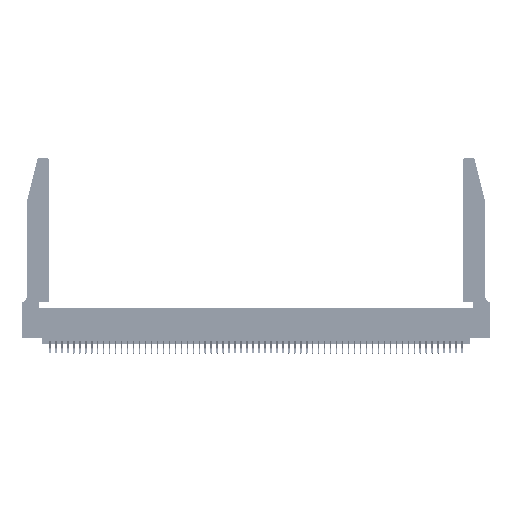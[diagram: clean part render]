
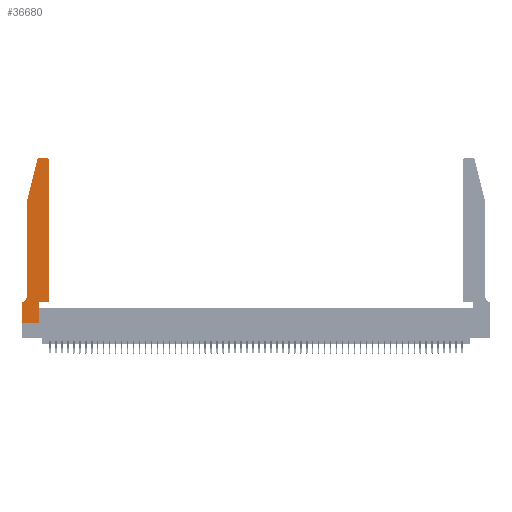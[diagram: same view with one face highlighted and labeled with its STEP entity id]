
A CAD part, top view. The second image highlights one B-rep face of the part: STEP entity #36680.
In plain terms, the highlighted planar face has unit normal (0, 0, 1).
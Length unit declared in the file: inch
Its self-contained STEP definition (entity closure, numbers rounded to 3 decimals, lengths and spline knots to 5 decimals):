
#419 = LINE ( 'NONE', #42385, #19449 ) ;
#731 = VERTEX_POINT ( 'NONE', #7288 ) ;
#1099 = CARTESIAN_POINT ( 'NONE',  ( 0.2865, 0.35, 0.37 ) ) ;
#2258 = LINE ( 'NONE', #23339, #9062 ) ;
#2402 = VERTEX_POINT ( 'NONE', #34915 ) ;
#2714 = CARTESIAN_POINT ( 'NONE',  ( 0.4205, 2.72, 0.37 ) ) ;
#3267 = EDGE_LOOP ( 'NONE', ( #22758, #41664, #4984, #45784, #14533, #25274, #8740, #31765, #51110, #8855, #9467, #22605 ) ) ;
#3878 = VECTOR ( 'NONE', #18521, 39.37008 ) ;
#4937 = LINE ( 'NONE', #1099, #11711 ) ;
#4984 = ORIENTED_EDGE ( 'NONE', *, *, #9804, .T. ) ;
#5143 = EDGE_CURVE ( 'NONE', #15108, #14876, #2258, .T. ) ;
#5638 = LINE ( 'NONE', #22326, #36915 ) ;
#5743 = EDGE_CURVE ( 'NONE', #42289, #31634, #5638, .T. ) ;
#6304 = AXIS2_PLACEMENT_3D ( 'NONE', #19725, #20277, #24291 ) ;
#7288 = CARTESIAN_POINT ( 'NONE',  ( 0.4505, 2.72, 0.37 ) ) ;
#7541 = DIRECTION ( 'NONE',  ( -0.239, -0.971, 0. ) ) ;
#7626 = CARTESIAN_POINT ( 'NONE',  ( 0.2865, 0., 0.37 ) ) ;
#7934 = AXIS2_PLACEMENT_3D ( 'NONE', #2714, #42114, #54968 ) ;
#8740 = ORIENTED_EDGE ( 'NONE', *, *, #15835, .T. ) ;
#8855 = ORIENTED_EDGE ( 'NONE', *, *, #5743, .T. ) ;
#9062 = VECTOR ( 'NONE', #10941, 39.37008 ) ;
#9467 = ORIENTED_EDGE ( 'NONE', *, *, #48293, .T. ) ;
#9804 = EDGE_CURVE ( 'NONE', #19901, #2402, #419, .T. ) ;
#10338 = DIRECTION ( 'NONE',  ( 1., 0., 0. ) ) ;
#10941 = DIRECTION ( 'NONE',  ( 1., 0., 0. ) ) ;
#11181 = EDGE_CURVE ( 'NONE', #46475, #19901, #34930, .T. ) ;
#11704 = DIRECTION ( 'NONE',  ( -1., 0., 0. ) ) ;
#11711 = VECTOR ( 'NONE', #35891, 39.37008 ) ;
#12012 = VERTEX_POINT ( 'NONE', #38476 ) ;
#12466 = VERTEX_POINT ( 'NONE', #49826 ) ;
#14117 = EDGE_CURVE ( 'NONE', #2402, #12466, #52346, .T. ) ;
#14159 = CARTESIAN_POINT ( 'NONE',  ( 0.2865, 0.35, 0.37 ) ) ;
#14345 = AXIS2_PLACEMENT_3D ( 'NONE', #31004, #39820, #30823 ) ;
#14533 = ORIENTED_EDGE ( 'NONE', *, *, #25234, .T. ) ;
#14876 = VERTEX_POINT ( 'NONE', #7626 ) ;
#15108 = VERTEX_POINT ( 'NONE', #22956 ) ;
#15835 = EDGE_CURVE ( 'NONE', #33642, #15108, #26275, .T. ) ;
#15931 = CARTESIAN_POINT ( 'NONE',  ( 0.2605, 2.75, 0.37 ) ) ;
#18521 = DIRECTION ( 'NONE',  ( 0., -1., 0. ) ) ;
#19337 = LINE ( 'NONE', #44659, #52683 ) ;
#19449 = VECTOR ( 'NONE', #7541, 39.37008 ) ;
#19725 = CARTESIAN_POINT ( 'NONE',  ( 0.284, 2.72, 0.37 ) ) ;
#19869 = VECTOR ( 'NONE', #54717, 39.37008 ) ;
#19901 = VERTEX_POINT ( 'NONE', #21024 ) ;
#20277 = DIRECTION ( 'NONE',  ( 0., 0., 1. ) ) ;
#21024 = CARTESIAN_POINT ( 'NONE',  ( 0.25487, 2.72718, 0.37 ) ) ;
#22088 = CARTESIAN_POINT ( 'NONE',  ( 0.0755, 2., 0.37 ) ) ;
#22326 = CARTESIAN_POINT ( 'NONE',  ( 0.4505, 0.35, 0.37 ) ) ;
#22493 = CARTESIAN_POINT ( 'NONE',  ( 0.0055, 0.35, 0.37 ) ) ;
#22605 = ORIENTED_EDGE ( 'NONE', *, *, #52879, .T. ) ;
#22758 = ORIENTED_EDGE ( 'NONE', *, *, #40502, .T. ) ;
#22887 = VERTEX_POINT ( 'NONE', #22493 ) ;
#22956 = CARTESIAN_POINT ( 'NONE',  ( 0., 0., 0.37 ) ) ;
#23282 = CARTESIAN_POINT ( 'NONE',  ( 0., 0.35, 0.37 ) ) ;
#23339 = CARTESIAN_POINT ( 'NONE',  ( 0., 0., 0.37 ) ) ;
#23662 = DIRECTION ( 'NONE',  ( 1., 0., 0. ) ) ;
#24291 = DIRECTION ( 'NONE',  ( 1., 0., 0. ) ) ;
#25234 = EDGE_CURVE ( 'NONE', #12466, #22887, #53237, .T. ) ;
#25274 = ORIENTED_EDGE ( 'NONE', *, *, #40765, .T. ) ;
#26137 = CARTESIAN_POINT ( 'NONE',  ( 0., 0.35, 0.37 ) ) ;
#26275 = LINE ( 'NONE', #49121, #3878 ) ;
#27408 = CIRCLE ( 'NONE', #7934, 0.03 ) ;
#27488 = VECTOR ( 'NONE', #11704, 39.37008 ) ;
#28793 = CARTESIAN_POINT ( 'NONE',  ( 0.284, 2.75, 0.37 ) ) ;
#30823 = DIRECTION ( 'NONE',  ( -1., 0., 0. ) ) ;
#31004 = CARTESIAN_POINT ( 'NONE',  ( 0.0055, 0.42, 0.37 ) ) ;
#31397 = LINE ( 'NONE', #50723, #19869 ) ;
#31634 = VERTEX_POINT ( 'NONE', #31699 ) ;
#31699 = CARTESIAN_POINT ( 'NONE',  ( 0.4505, 0.35, 0.37 ) ) ;
#31765 = ORIENTED_EDGE ( 'NONE', *, *, #5143, .T. ) ;
#33642 = VERTEX_POINT ( 'NONE', #26137 ) ;
#34915 = CARTESIAN_POINT ( 'NONE',  ( 0.0755, 2., 0.37 ) ) ;
#34930 = CIRCLE ( 'NONE', #6304, 0.03 ) ;
#35891 = DIRECTION ( 'NONE',  ( 0., 1., 0. ) ) ;
#36068 = DIRECTION ( 'NONE',  ( -1., 0., 0. ) ) ;
#36680 = ADVANCED_FACE ( 'NONE', ( #41566 ), #53527, .T. ) ;
#36915 = VECTOR ( 'NONE', #23662, 39.37008 ) ;
#38476 = CARTESIAN_POINT ( 'NONE',  ( 0.4205, 2.75, 0.37 ) ) ;
#39820 = DIRECTION ( 'NONE',  ( 0., 0., -1. ) ) ;
#40502 = EDGE_CURVE ( 'NONE', #12012, #46475, #49281, .T. ) ;
#40765 = EDGE_CURVE ( 'NONE', #22887, #33642, #19337, .T. ) ;
#41025 = DIRECTION ( 'NONE',  ( 0., 0., 1. ) ) ;
#41566 = FACE_OUTER_BOUND ( 'NONE', #3267, .T. ) ;
#41664 = ORIENTED_EDGE ( 'NONE', *, *, #11181, .T. ) ;
#42114 = DIRECTION ( 'NONE',  ( 0., 0., 1. ) ) ;
#42289 = VERTEX_POINT ( 'NONE', #14159 ) ;
#42385 = CARTESIAN_POINT ( 'NONE',  ( 0.0755, 2., 0.37 ) ) ;
#44659 = CARTESIAN_POINT ( 'NONE',  ( 0.0755, 0.35, 0.37 ) ) ;
#45784 = ORIENTED_EDGE ( 'NONE', *, *, #14117, .T. ) ;
#46475 = VERTEX_POINT ( 'NONE', #28793 ) ;
#47998 = EDGE_CURVE ( 'NONE', #14876, #42289, #4937, .T. ) ;
#48293 = EDGE_CURVE ( 'NONE', #31634, #731, #31397, .T. ) ;
#49121 = CARTESIAN_POINT ( 'NONE',  ( 0., 0., 0.37 ) ) ;
#49281 = LINE ( 'NONE', #15931, #27488 ) ;
#49826 = CARTESIAN_POINT ( 'NONE',  ( 0.0755, 0.42, 0.37 ) ) ;
#50723 = CARTESIAN_POINT ( 'NONE',  ( 0.4505, 0.35, 0.37 ) ) ;
#51110 = ORIENTED_EDGE ( 'NONE', *, *, #47998, .T. ) ;
#51916 = AXIS2_PLACEMENT_3D ( 'NONE', #23282, #41025, #10338 ) ;
#52346 = LINE ( 'NONE', #22088, #55067 ) ;
#52527 = DIRECTION ( 'NONE',  ( 0., -1., 0. ) ) ;
#52683 = VECTOR ( 'NONE', #36068, 39.37008 ) ;
#52879 = EDGE_CURVE ( 'NONE', #731, #12012, #27408, .T. ) ;
#53237 = CIRCLE ( 'NONE', #14345, 0.07 ) ;
#53527 = PLANE ( 'NONE',  #51916 ) ;
#54717 = DIRECTION ( 'NONE',  ( 0., 1., 0. ) ) ;
#54968 = DIRECTION ( 'NONE',  ( 1., 0., 0. ) ) ;
#55067 = VECTOR ( 'NONE', #52527, 39.37008 ) ;
